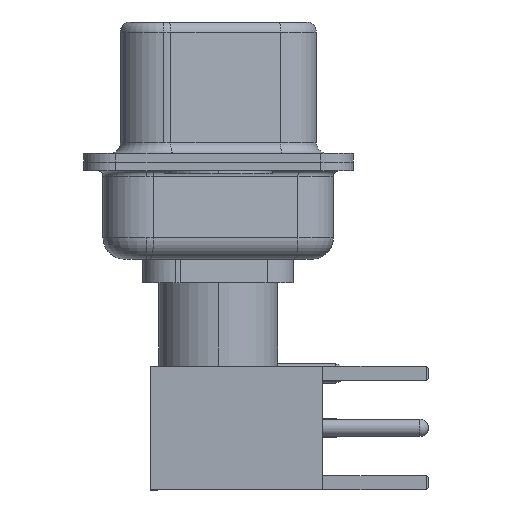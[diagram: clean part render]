
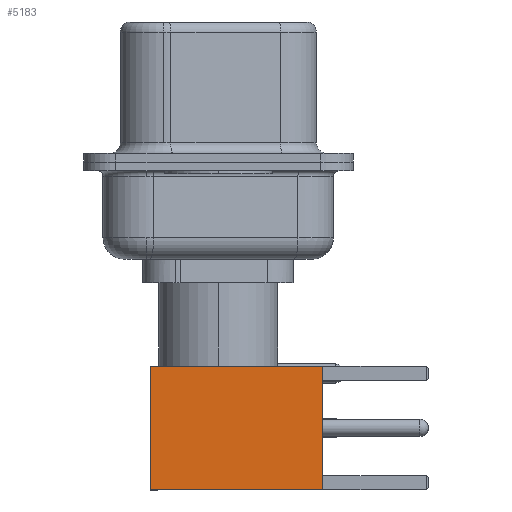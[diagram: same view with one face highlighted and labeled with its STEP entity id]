
A CAD part, left-side view. The second image highlights one B-rep face of the part: STEP entity #5183.
In plain terms, the highlighted face is planar.
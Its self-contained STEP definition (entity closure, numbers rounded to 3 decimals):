
#1088 = CARTESIAN_POINT ( 'NONE',  ( 0., 2.875, 0. ) ) ;
#2254 = CARTESIAN_POINT ( 'NONE',  ( 2.875, 2.875, 8. ) ) ;
#2800 = AXIS2_PLACEMENT_3D ( 'NONE', #3363, #21091, #23284 ) ;
#3363 = CARTESIAN_POINT ( 'NONE',  ( 2.875, 2.875, 0. ) ) ;
#3610 = CARTESIAN_POINT ( 'NONE',  ( -2.875, 2.875, 0. ) ) ;
#4656 = CARTESIAN_POINT ( 'NONE',  ( -2.875, 2.875, 0. ) ) ;
#4991 = LINE ( 'NONE', #17150, #13814 ) ;
#5183 = ADVANCED_FACE ( 'NONE', ( #21603 ), #23037, .T. ) ;
#5292 = CARTESIAN_POINT ( 'NONE',  ( 0., 2.875, 8. ) ) ;
#5548 = LINE ( 'NONE', #5292, #23518 ) ;
#5732 = CARTESIAN_POINT ( 'NONE',  ( -2.875, 2.875, 8. ) ) ;
#5859 = VECTOR ( 'NONE', #18543, 1000. ) ;
#5879 = ORIENTED_EDGE ( 'NONE', *, *, #8783, .F. ) ;
#8783 = EDGE_CURVE ( 'NONE', #21327, #12723, #5548, .T. ) ;
#8997 = DIRECTION ( 'NONE',  ( 0., 0., -1. ) ) ;
#10561 = ORIENTED_EDGE ( 'NONE', *, *, #13089, .T. ) ;
#11237 = EDGE_LOOP ( 'NONE', ( #21477, #10561, #15991, #5879 ) ) ;
#12723 = VERTEX_POINT ( 'NONE', #5732 ) ;
#13089 = EDGE_CURVE ( 'NONE', #17696, #23467, #13439, .T. ) ;
#13439 = LINE ( 'NONE', #1088, #5859 ) ;
#13814 = VECTOR ( 'NONE', #8997, 1000. ) ;
#13983 = LINE ( 'NONE', #4656, #23525 ) ;
#15166 = EDGE_CURVE ( 'NONE', #21327, #17696, #4991, .T. ) ;
#15382 = DIRECTION ( 'NONE',  ( -1., 0., 0. ) ) ;
#15991 = ORIENTED_EDGE ( 'NONE', *, *, #21789, .F. ) ;
#16308 = DIRECTION ( 'NONE',  ( 0., 0., -1. ) ) ;
#17150 = CARTESIAN_POINT ( 'NONE',  ( 2.875, 2.875, 0. ) ) ;
#17696 = VERTEX_POINT ( 'NONE', #21348 ) ;
#18543 = DIRECTION ( 'NONE',  ( -1., 0., 0. ) ) ;
#21091 = DIRECTION ( 'NONE',  ( 0., 1., 0. ) ) ;
#21327 = VERTEX_POINT ( 'NONE', #2254 ) ;
#21348 = CARTESIAN_POINT ( 'NONE',  ( 2.875, 2.875, 0. ) ) ;
#21477 = ORIENTED_EDGE ( 'NONE', *, *, #15166, .T. ) ;
#21603 = FACE_OUTER_BOUND ( 'NONE', #11237, .T. ) ;
#21789 = EDGE_CURVE ( 'NONE', #12723, #23467, #13983, .T. ) ;
#23037 = PLANE ( 'NONE',  #2800 ) ;
#23284 = DIRECTION ( 'NONE',  ( 0., 0., 1. ) ) ;
#23467 = VERTEX_POINT ( 'NONE', #3610 ) ;
#23518 = VECTOR ( 'NONE', #15382, 1000. ) ;
#23525 = VECTOR ( 'NONE', #16308, 1000. ) ;
